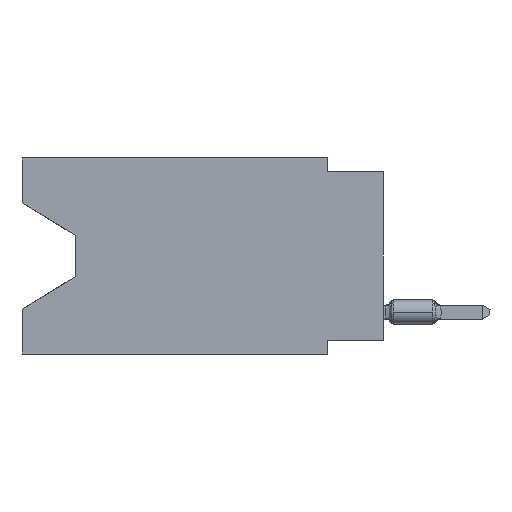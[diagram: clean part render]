
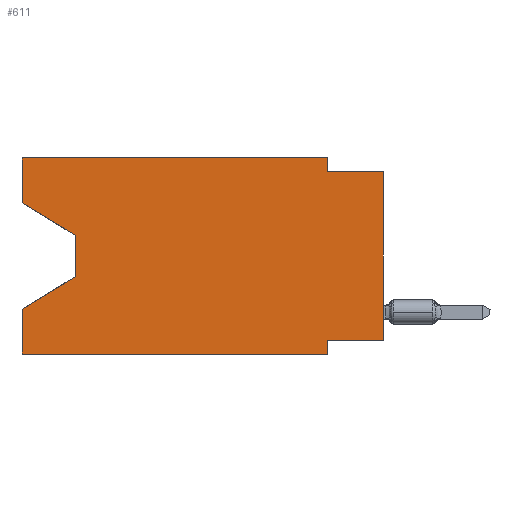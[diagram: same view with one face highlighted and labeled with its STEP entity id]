
A CAD part, left-side view. The second image highlights one B-rep face of the part: STEP entity #611.
In plain terms, the highlighted planar face has unit normal (-1, 0, 0).
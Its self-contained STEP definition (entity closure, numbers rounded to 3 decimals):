
#178 = CARTESIAN_POINT ( 'NONE',  ( 0., 2.54, -8.89 ) ) ;
#498 = CARTESIAN_POINT ( 'NONE',  ( 0., 2.54, 0. ) ) ;
#611 = ADVANCED_FACE ( 'NONE', ( #10306 ), #31710, .F. ) ;
#716 = CARTESIAN_POINT ( 'NONE',  ( 0., 0., -0.635 ) ) ;
#918 = DIRECTION ( 'NONE',  ( 0., 0., 1. ) ) ;
#1037 = ORIENTED_EDGE ( 'NONE', *, *, #8673, .F. ) ;
#1691 = EDGE_CURVE ( 'NONE', #19219, #11872, #15411, .T. ) ;
#2336 = ORIENTED_EDGE ( 'NONE', *, *, #9614, .F. ) ;
#2730 = CARTESIAN_POINT ( 'NONE',  ( 0., 13.97, -3.505 ) ) ;
#2888 = DIRECTION ( 'NONE',  ( 0., 0., 1. ) ) ;
#3041 = VECTOR ( 'NONE', #918, 1000. ) ;
#3804 = DIRECTION ( 'NONE',  ( 0., -1., 0. ) ) ;
#4164 = ORIENTED_EDGE ( 'NONE', *, *, #4279, .F. ) ;
#4216 = CARTESIAN_POINT ( 'NONE',  ( 0., 0., -0.635 ) ) ;
#4279 = EDGE_CURVE ( 'NONE', #33387, #23753, #24882, .T. ) ;
#4373 = LINE ( 'NONE', #4216, #28071 ) ;
#4433 = VECTOR ( 'NONE', #20922, 1000. ) ;
#4841 = CARTESIAN_POINT ( 'NONE',  ( 0., 16.383, -8.89 ) ) ;
#5042 = VERTEX_POINT ( 'NONE', #19827 ) ;
#6423 = DIRECTION ( 'NONE',  ( 0., -1., 0. ) ) ;
#6486 = EDGE_CURVE ( 'NONE', #14187, #30232, #7741, .T. ) ;
#7741 = LINE ( 'NONE', #33583, #9427 ) ;
#8017 = VECTOR ( 'NONE', #31747, 1000. ) ;
#8293 = VERTEX_POINT ( 'NONE', #716 ) ;
#8557 = VERTEX_POINT ( 'NONE', #178 ) ;
#8673 = EDGE_CURVE ( 'NONE', #14187, #33387, #26171, .T. ) ;
#8827 = CARTESIAN_POINT ( 'NONE',  ( 0., 16.383, 0. ) ) ;
#9427 = VECTOR ( 'NONE', #33411, 1000. ) ;
#9458 = VECTOR ( 'NONE', #23005, 1000. ) ;
#9614 = EDGE_CURVE ( 'NONE', #17792, #17151, #30617, .T. ) ;
#10306 = FACE_OUTER_BOUND ( 'NONE', #13559, .T. ) ;
#10961 = EDGE_CURVE ( 'NONE', #30232, #5042, #15650, .T. ) ;
#11030 = AXIS2_PLACEMENT_3D ( 'NONE', #18302, #25780, #23738 ) ;
#11337 = CARTESIAN_POINT ( 'NONE',  ( 0., 16.383, -2.038 ) ) ;
#11660 = EDGE_CURVE ( 'NONE', #30735, #8293, #4373, .T. ) ;
#11872 = VERTEX_POINT ( 'NONE', #18969 ) ;
#12477 = LINE ( 'NONE', #12643, #9458 ) ;
#12643 = CARTESIAN_POINT ( 'NONE',  ( 0., 2.54, -8.89 ) ) ;
#12662 = EDGE_CURVE ( 'NONE', #23753, #30735, #23781, .T. ) ;
#12885 = DIRECTION ( 'NONE',  ( 0., 1., 0. ) ) ;
#13559 = EDGE_LOOP ( 'NONE', ( #21192, #32784, #27761, #2336, #23251, #17967, #26980, #16582, #30597, #32589, #4164, #1037 ) ) ;
#13632 = CARTESIAN_POINT ( 'NONE',  ( 0., 13.97, -3.505 ) ) ;
#14187 = VERTEX_POINT ( 'NONE', #11337 ) ;
#15250 = VECTOR ( 'NONE', #2888, 1000. ) ;
#15411 = LINE ( 'NONE', #25786, #23011 ) ;
#15650 = LINE ( 'NONE', #2730, #4433 ) ;
#15959 = EDGE_CURVE ( 'NONE', #5042, #17151, #31576, .T. ) ;
#16361 = LINE ( 'NONE', #16866, #3041 ) ;
#16450 = DIRECTION ( 'NONE',  ( 0., 0., -1. ) ) ;
#16582 = ORIENTED_EDGE ( 'NONE', *, *, #16926, .T. ) ;
#16851 = CARTESIAN_POINT ( 'NONE',  ( 0., 16.383, 0. ) ) ;
#16866 = CARTESIAN_POINT ( 'NONE',  ( 0., 0., 0. ) ) ;
#16926 = EDGE_CURVE ( 'NONE', #19219, #8293, #16361, .T. ) ;
#17151 = VERTEX_POINT ( 'NONE', #26191 ) ;
#17792 = VERTEX_POINT ( 'NONE', #4841 ) ;
#17967 = ORIENTED_EDGE ( 'NONE', *, *, #26479, .F. ) ;
#18302 = CARTESIAN_POINT ( 'NONE',  ( 0., 16.383, 0. ) ) ;
#18969 = CARTESIAN_POINT ( 'NONE',  ( 0., 2.54, -8.255 ) ) ;
#19219 = VERTEX_POINT ( 'NONE', #31882 ) ;
#19827 = CARTESIAN_POINT ( 'NONE',  ( 0., 13.97, -5.385 ) ) ;
#20922 = DIRECTION ( 'NONE',  ( 0., 0., -1. ) ) ;
#21192 = ORIENTED_EDGE ( 'NONE', *, *, #6486, .T. ) ;
#21384 = CARTESIAN_POINT ( 'NONE',  ( 0., 13.97, -5.385 ) ) ;
#23005 = DIRECTION ( 'NONE',  ( 0., 0., -1. ) ) ;
#23011 = VECTOR ( 'NONE', #12885, 1000. ) ;
#23251 = ORIENTED_EDGE ( 'NONE', *, *, #24913, .T. ) ;
#23738 = DIRECTION ( 'NONE',  ( 0., 0., -1. ) ) ;
#23753 = VERTEX_POINT ( 'NONE', #26541 ) ;
#23781 = LINE ( 'NONE', #498, #24287 ) ;
#24287 = VECTOR ( 'NONE', #16450, 1000. ) ;
#24830 = CARTESIAN_POINT ( 'NONE',  ( 0., 16.383, 0. ) ) ;
#24882 = LINE ( 'NONE', #27094, #26700 ) ;
#24913 = EDGE_CURVE ( 'NONE', #17792, #8557, #25758, .T. ) ;
#25658 = VECTOR ( 'NONE', #28654, 1000. ) ;
#25758 = LINE ( 'NONE', #26247, #25658 ) ;
#25780 = DIRECTION ( 'NONE',  ( 1., 0., 0. ) ) ;
#25786 = CARTESIAN_POINT ( 'NONE',  ( 0., 0., -8.255 ) ) ;
#26171 = LINE ( 'NONE', #8827, #15250 ) ;
#26191 = CARTESIAN_POINT ( 'NONE',  ( 0., 16.383, -6.852 ) ) ;
#26247 = CARTESIAN_POINT ( 'NONE',  ( 0., 16.383, -8.89 ) ) ;
#26479 = EDGE_CURVE ( 'NONE', #11872, #8557, #12477, .T. ) ;
#26541 = CARTESIAN_POINT ( 'NONE',  ( 0., 2.54, 0. ) ) ;
#26700 = VECTOR ( 'NONE', #3804, 1000. ) ;
#26980 = ORIENTED_EDGE ( 'NONE', *, *, #1691, .F. ) ;
#27094 = CARTESIAN_POINT ( 'NONE',  ( 0., 16.383, 0. ) ) ;
#27184 = VECTOR ( 'NONE', #33157, 1000. ) ;
#27761 = ORIENTED_EDGE ( 'NONE', *, *, #15959, .T. ) ;
#28071 = VECTOR ( 'NONE', #6423, 1000. ) ;
#28654 = DIRECTION ( 'NONE',  ( 0., -1., 0. ) ) ;
#30232 = VERTEX_POINT ( 'NONE', #13632 ) ;
#30597 = ORIENTED_EDGE ( 'NONE', *, *, #11660, .F. ) ;
#30617 = LINE ( 'NONE', #16851, #27184 ) ;
#30735 = VERTEX_POINT ( 'NONE', #31955 ) ;
#31576 = LINE ( 'NONE', #21384, #8017 ) ;
#31710 = PLANE ( 'NONE',  #11030 ) ;
#31747 = DIRECTION ( 'NONE',  ( 0., 0.855, -0.519 ) ) ;
#31882 = CARTESIAN_POINT ( 'NONE',  ( 0., 0., -8.255 ) ) ;
#31955 = CARTESIAN_POINT ( 'NONE',  ( 0., 2.54, -0.635 ) ) ;
#32589 = ORIENTED_EDGE ( 'NONE', *, *, #12662, .F. ) ;
#32784 = ORIENTED_EDGE ( 'NONE', *, *, #10961, .T. ) ;
#33157 = DIRECTION ( 'NONE',  ( 0., 0., 1. ) ) ;
#33387 = VERTEX_POINT ( 'NONE', #24830 ) ;
#33411 = DIRECTION ( 'NONE',  ( 0., -0.855, -0.519 ) ) ;
#33583 = CARTESIAN_POINT ( 'NONE',  ( 0., 16.383, -2.038 ) ) ;
